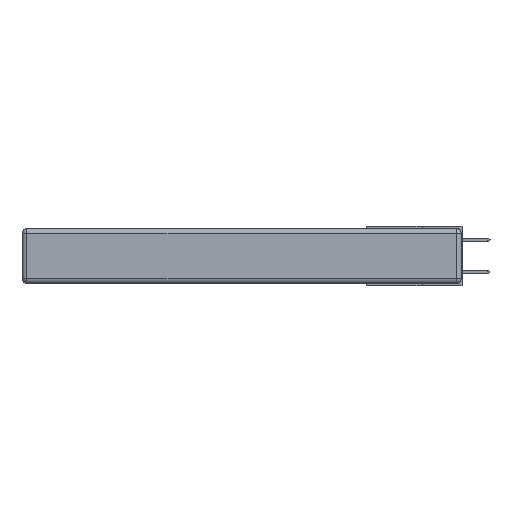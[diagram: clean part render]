
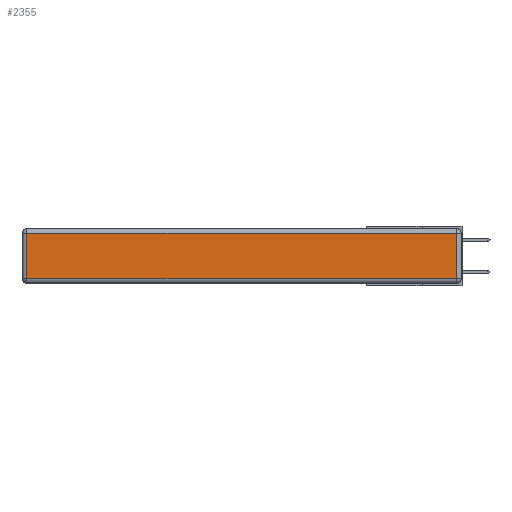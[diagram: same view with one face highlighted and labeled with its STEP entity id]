
A CAD part, left-side view. The second image highlights one B-rep face of the part: STEP entity #2355.
In plain terms, the highlighted planar face has unit normal (-1, 0, 0).
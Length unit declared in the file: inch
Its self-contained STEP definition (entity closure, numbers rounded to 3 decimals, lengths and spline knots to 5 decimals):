
#237 = CARTESIAN_POINT ( 'NONE',  ( 0., 0.03, -0.343 ) ) ;
#1312 = VECTOR ( 'NONE', #10807, 39.37008 ) ;
#1424 = CARTESIAN_POINT ( 'NONE',  ( 0., 0., -0.313 ) ) ;
#1900 = DIRECTION ( 'NONE',  ( 0., 0., 1. ) ) ;
#2061 = VERTEX_POINT ( 'NONE', #6375 ) ;
#2355 = ADVANCED_FACE ( 'NONE', ( #8529 ), #13980, .T. ) ;
#2918 = EDGE_LOOP ( 'NONE', ( #17427, #17854, #11425, #17173 ) ) ;
#3571 = CARTESIAN_POINT ( 'NONE',  ( 0., 2.72, -0.313 ) ) ;
#3716 = LINE ( 'NONE', #237, #20570 ) ;
#4439 = CARTESIAN_POINT ( 'NONE',  ( 0., 2.72, -0.343 ) ) ;
#5606 = EDGE_CURVE ( 'NONE', #20566, #16778, #15066, .T. ) ;
#6375 = CARTESIAN_POINT ( 'NONE',  ( 0., 0.03, -0.03 ) ) ;
#7474 = DIRECTION ( 'NONE',  ( -1., 0., 0. ) ) ;
#8529 = FACE_OUTER_BOUND ( 'NONE', #2918, .T. ) ;
#9095 = DIRECTION ( 'NONE',  ( 0., 0., 1. ) ) ;
#9191 = EDGE_CURVE ( 'NONE', #2061, #20027, #13435, .T. ) ;
#10705 = EDGE_CURVE ( 'NONE', #20027, #20566, #20756, .T. ) ;
#10807 = DIRECTION ( 'NONE',  ( 0., 0., -1. ) ) ;
#11425 = ORIENTED_EDGE ( 'NONE', *, *, #9191, .T. ) ;
#12125 = CARTESIAN_POINT ( 'NONE',  ( 0., 2.75, -0.03 ) ) ;
#12665 = VECTOR ( 'NONE', #18853, 39.37008 ) ;
#13435 = LINE ( 'NONE', #12125, #12665 ) ;
#13980 = PLANE ( 'NONE',  #15427 ) ;
#14256 = CARTESIAN_POINT ( 'NONE',  ( 0., 2.72, -0.03 ) ) ;
#15066 = LINE ( 'NONE', #1424, #19647 ) ;
#15427 = AXIS2_PLACEMENT_3D ( 'NONE', #15641, #7474, #9095 ) ;
#15641 = CARTESIAN_POINT ( 'NONE',  ( 0., 0., -0.343 ) ) ;
#15705 = EDGE_CURVE ( 'NONE', #16778, #2061, #3716, .T. ) ;
#16778 = VERTEX_POINT ( 'NONE', #21084 ) ;
#17173 = ORIENTED_EDGE ( 'NONE', *, *, #10705, .T. ) ;
#17427 = ORIENTED_EDGE ( 'NONE', *, *, #5606, .T. ) ;
#17854 = ORIENTED_EDGE ( 'NONE', *, *, #15705, .T. ) ;
#18853 = DIRECTION ( 'NONE',  ( 0., 1., 0. ) ) ;
#19458 = DIRECTION ( 'NONE',  ( 0., -1., 0. ) ) ;
#19647 = VECTOR ( 'NONE', #19458, 39.37008 ) ;
#20027 = VERTEX_POINT ( 'NONE', #14256 ) ;
#20566 = VERTEX_POINT ( 'NONE', #3571 ) ;
#20570 = VECTOR ( 'NONE', #1900, 39.37008 ) ;
#20756 = LINE ( 'NONE', #4439, #1312 ) ;
#21084 = CARTESIAN_POINT ( 'NONE',  ( 0., 0.03, -0.313 ) ) ;
